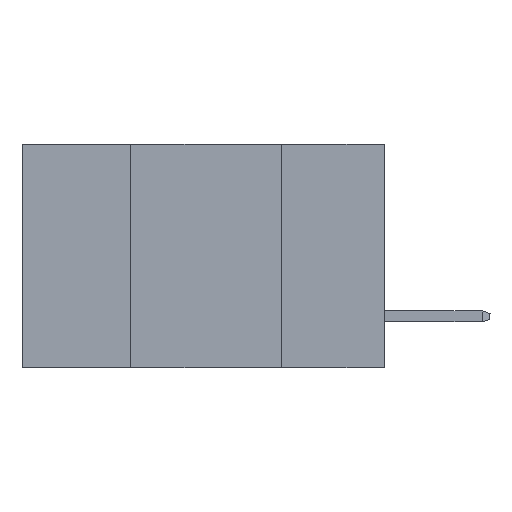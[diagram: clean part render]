
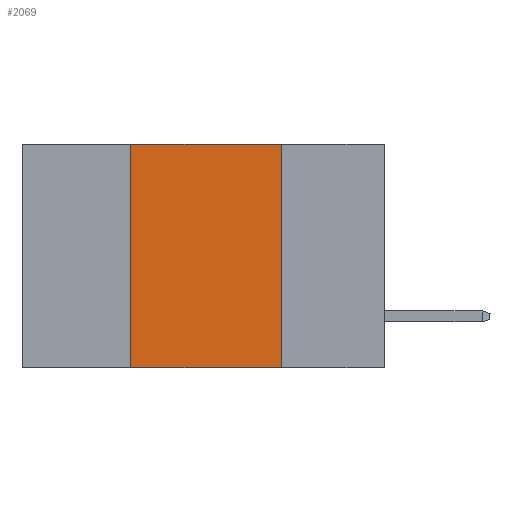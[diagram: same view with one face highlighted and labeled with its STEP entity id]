
A CAD part, left-side view. The second image highlights one B-rep face of the part: STEP entity #2069.
In plain terms, the highlighted planar face has unit normal (-1, 0, 0).
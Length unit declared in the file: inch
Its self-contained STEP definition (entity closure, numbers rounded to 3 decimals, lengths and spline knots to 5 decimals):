
#422 = ORIENTED_EDGE ( 'NONE', *, *, #6916, .T. ) ;
#584 = VERTEX_POINT ( 'NONE', #3925 ) ;
#1375 = DIRECTION ( 'NONE',  ( 0., -1., 0. ) ) ;
#1477 = VERTEX_POINT ( 'NONE', #9999 ) ;
#1787 = DIRECTION ( 'NONE',  ( 0., 0., 1. ) ) ;
#1930 = CARTESIAN_POINT ( 'NONE',  ( 0., 0.42, -0.37 ) ) ;
#2069 = ADVANCED_FACE ( 'NONE', ( #6371 ), #10325, .F. ) ;
#3300 = VECTOR ( 'NONE', #8767, 39.37008 ) ;
#3779 = CARTESIAN_POINT ( 'NONE',  ( 0., 0.17, -0.37 ) ) ;
#3867 = VERTEX_POINT ( 'NONE', #1930 ) ;
#3917 = CARTESIAN_POINT ( 'NONE',  ( 0., 0.6, -0.37 ) ) ;
#3925 = CARTESIAN_POINT ( 'NONE',  ( 0., 0.17, -0.37 ) ) ;
#4127 = EDGE_CURVE ( 'NONE', #1477, #9730, #5510, .T. ) ;
#4885 = VECTOR ( 'NONE', #8969, 39.37008 ) ;
#5510 = LINE ( 'NONE', #12410, #10894 ) ;
#5581 = EDGE_LOOP ( 'NONE', ( #6502, #10226, #10908, #422 ) ) ;
#6371 = FACE_OUTER_BOUND ( 'NONE', #5581, .T. ) ;
#6502 = ORIENTED_EDGE ( 'NONE', *, *, #12209, .F. ) ;
#6916 = EDGE_CURVE ( 'NONE', #3867, #584, #9889, .T. ) ;
#8360 = DIRECTION ( 'NONE',  ( 1., 0., 0. ) ) ;
#8767 = DIRECTION ( 'NONE',  ( 0., 0., -1. ) ) ;
#8969 = DIRECTION ( 'NONE',  ( 0., -1., 0. ) ) ;
#9730 = VERTEX_POINT ( 'NONE', #10334 ) ;
#9762 = AXIS2_PLACEMENT_3D ( 'NONE', #11395, #8360, #12356 ) ;
#9889 = LINE ( 'NONE', #3917, #4885 ) ;
#9999 = CARTESIAN_POINT ( 'NONE',  ( 0., 0.42, 0. ) ) ;
#10226 = ORIENTED_EDGE ( 'NONE', *, *, #4127, .F. ) ;
#10325 = PLANE ( 'NONE',  #9762 ) ;
#10334 = CARTESIAN_POINT ( 'NONE',  ( 0., 0.17, 0. ) ) ;
#10722 = LINE ( 'NONE', #10859, #11029 ) ;
#10859 = CARTESIAN_POINT ( 'NONE',  ( 0., 0.42, -0.37 ) ) ;
#10894 = VECTOR ( 'NONE', #1375, 39.37008 ) ;
#10908 = ORIENTED_EDGE ( 'NONE', *, *, #12786, .F. ) ;
#11029 = VECTOR ( 'NONE', #1787, 39.37008 ) ;
#11395 = CARTESIAN_POINT ( 'NONE',  ( 0., 0.6, 0. ) ) ;
#12209 = EDGE_CURVE ( 'NONE', #9730, #584, #12631, .T. ) ;
#12356 = DIRECTION ( 'NONE',  ( 0., 0., -1. ) ) ;
#12410 = CARTESIAN_POINT ( 'NONE',  ( 0., 0.6, 0. ) ) ;
#12631 = LINE ( 'NONE', #3779, #3300 ) ;
#12786 = EDGE_CURVE ( 'NONE', #3867, #1477, #10722, .T. ) ;
